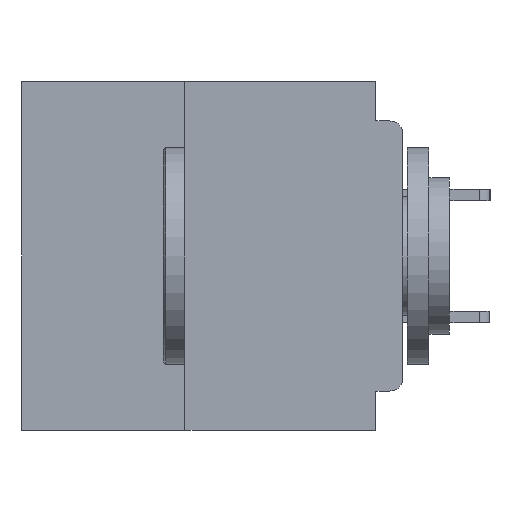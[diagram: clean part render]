
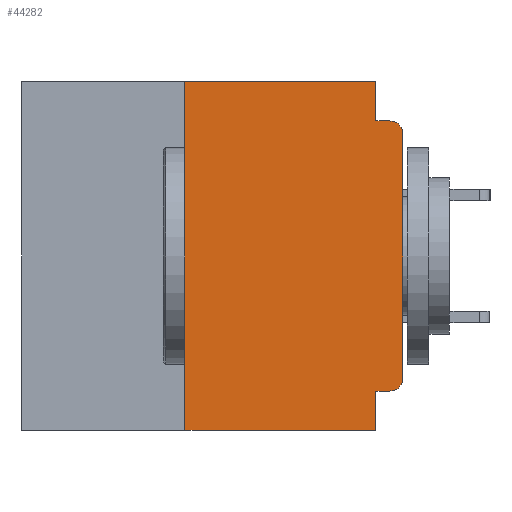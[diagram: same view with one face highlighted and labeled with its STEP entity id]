
A CAD part, left-side view. The second image highlights one B-rep face of the part: STEP entity #44282.
In plain terms, the highlighted planar face has unit normal (-1, 0, 0).
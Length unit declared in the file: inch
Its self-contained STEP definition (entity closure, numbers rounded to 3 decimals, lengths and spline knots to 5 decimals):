
#142 = CARTESIAN_POINT ( 'NONE',  ( 0., 0.031, -0.4 ) ) ;
#254 = CARTESIAN_POINT ( 'NONE',  ( 0., 0., -0.355 ) ) ;
#1671 = VECTOR ( 'NONE', #31259, 39.37008 ) ;
#1722 = LINE ( 'NONE', #44877, #25280 ) ;
#1834 = ORIENTED_EDGE ( 'NONE', *, *, #27117, .F. ) ;
#2905 = DIRECTION ( 'NONE',  ( -1., 0., 0. ) ) ;
#3507 = LINE ( 'NONE', #12196, #28640 ) ;
#3594 = CARTESIAN_POINT ( 'NONE',  ( 0., 0., 0. ) ) ;
#4801 = LINE ( 'NONE', #56178, #1671 ) ;
#7095 = CARTESIAN_POINT ( 'NONE',  ( 0., 0., -0.045 ) ) ;
#7521 = DIRECTION ( 'NONE',  ( 0., -1., 0. ) ) ;
#10218 = VERTEX_POINT ( 'NONE', #39901 ) ;
#11951 = ORIENTED_EDGE ( 'NONE', *, *, #59391, .T. ) ;
#12120 = LINE ( 'NONE', #20560, #50505 ) ;
#12196 = CARTESIAN_POINT ( 'NONE',  ( 0., 0.031, -0.4 ) ) ;
#12401 = CIRCLE ( 'NONE', #51283, 0.015 ) ;
#14349 = EDGE_CURVE ( 'NONE', #18761, #63500, #1722, .T. ) ;
#15446 = DIRECTION ( 'NONE',  ( 1., 0., 0. ) ) ;
#15535 = DIRECTION ( 'NONE',  ( 0., -1., 0. ) ) ;
#16565 = ORIENTED_EDGE ( 'NONE', *, *, #52209, .T. ) ;
#17229 = DIRECTION ( 'NONE',  ( 0., -1., 0. ) ) ;
#17236 = DIRECTION ( 'NONE',  ( 0., 0., -1. ) ) ;
#17350 = CIRCLE ( 'NONE', #60182, 0.015 ) ;
#17466 = FACE_OUTER_BOUND ( 'NONE', #23378, .T. ) ;
#18075 = VERTEX_POINT ( 'NONE', #24660 ) ;
#18497 = VECTOR ( 'NONE', #17229, 39.37008 ) ;
#18761 = VERTEX_POINT ( 'NONE', #25858 ) ;
#19036 = CARTESIAN_POINT ( 'NONE',  ( 0., 0., -0.34 ) ) ;
#20560 = CARTESIAN_POINT ( 'NONE',  ( 0., 0.437, -0.4 ) ) ;
#21001 = CARTESIAN_POINT ( 'NONE',  ( 0., 0.015, -0.06 ) ) ;
#22813 = VERTEX_POINT ( 'NONE', #32500 ) ;
#23378 = EDGE_LOOP ( 'NONE', ( #39533, #40731, #53599, #49705, #42236, #1834, #11951, #56199, #43870, #16565 ) ) ;
#24660 = CARTESIAN_POINT ( 'NONE',  ( 0., 0.25, -0.4 ) ) ;
#24862 = EDGE_CURVE ( 'NONE', #63500, #22813, #33412, .T. ) ;
#25280 = VECTOR ( 'NONE', #29947, 39.37008 ) ;
#25689 = CARTESIAN_POINT ( 'NONE',  ( 0., 0., -0.06 ) ) ;
#25858 = CARTESIAN_POINT ( 'NONE',  ( 0., 0.031, 0. ) ) ;
#26053 = DIRECTION ( 'NONE',  ( 0., 0., -1. ) ) ;
#26804 = CARTESIAN_POINT ( 'NONE',  ( 0., 0.25, 0. ) ) ;
#27117 = EDGE_CURVE ( 'NONE', #18075, #57961, #4801, .T. ) ;
#28640 = VECTOR ( 'NONE', #17236, 39.37008 ) ;
#28821 = DIRECTION ( 'NONE',  ( 0., 0., 1. ) ) ;
#29947 = DIRECTION ( 'NONE',  ( 0., 0., -1. ) ) ;
#31259 = DIRECTION ( 'NONE',  ( 0., 0., 1. ) ) ;
#31350 = VERTEX_POINT ( 'NONE', #19036 ) ;
#31920 = EDGE_CURVE ( 'NONE', #31350, #52558, #50338, .T. ) ;
#32500 = CARTESIAN_POINT ( 'NONE',  ( 0., 0.015, -0.045 ) ) ;
#32507 = CARTESIAN_POINT ( 'NONE',  ( 0., 0.437, 0. ) ) ;
#32633 = VERTEX_POINT ( 'NONE', #54981 ) ;
#32656 = EDGE_CURVE ( 'NONE', #10218, #32633, #59577, .T. ) ;
#32967 = CARTESIAN_POINT ( 'NONE',  ( 0., 0.015, -0.34 ) ) ;
#33412 = LINE ( 'NONE', #7095, #18497 ) ;
#34037 = VECTOR ( 'NONE', #7521, 39.37008 ) ;
#35377 = PLANE ( 'NONE',  #48294 ) ;
#37018 = VECTOR ( 'NONE', #28821, 39.37008 ) ;
#37120 = EDGE_CURVE ( 'NONE', #32633, #58378, #3507, .T. ) ;
#38001 = DIRECTION ( 'NONE',  ( 0., 0., -1. ) ) ;
#39533 = ORIENTED_EDGE ( 'NONE', *, *, #31920, .T. ) ;
#39901 = CARTESIAN_POINT ( 'NONE',  ( 0., 0.015, -0.355 ) ) ;
#40153 = EDGE_CURVE ( 'NONE', #52558, #22813, #17350, .T. ) ;
#40441 = CARTESIAN_POINT ( 'NONE',  ( 0., 0.437, 0. ) ) ;
#40731 = ORIENTED_EDGE ( 'NONE', *, *, #40153, .T. ) ;
#42236 = ORIENTED_EDGE ( 'NONE', *, *, #64357, .F. ) ;
#43870 = ORIENTED_EDGE ( 'NONE', *, *, #32656, .F. ) ;
#44282 = ADVANCED_FACE ( 'NONE', ( #17466 ), #35377, .F. ) ;
#44877 = CARTESIAN_POINT ( 'NONE',  ( 0., 0.031, 0. ) ) ;
#45426 = DIRECTION ( 'NONE',  ( 0., 1., 0. ) ) ;
#48294 = AXIS2_PLACEMENT_3D ( 'NONE', #40441, #15446, #50481 ) ;
#49705 = ORIENTED_EDGE ( 'NONE', *, *, #14349, .F. ) ;
#50338 = LINE ( 'NONE', #3594, #37018 ) ;
#50481 = DIRECTION ( 'NONE',  ( 0., 0., -1. ) ) ;
#50505 = VECTOR ( 'NONE', #15535, 39.37008 ) ;
#51283 = AXIS2_PLACEMENT_3D ( 'NONE', #32967, #2905, #38001 ) ;
#52209 = EDGE_CURVE ( 'NONE', #10218, #31350, #12401, .T. ) ;
#52558 = VERTEX_POINT ( 'NONE', #25689 ) ;
#53599 = ORIENTED_EDGE ( 'NONE', *, *, #24862, .F. ) ;
#54981 = CARTESIAN_POINT ( 'NONE',  ( 0., 0.031, -0.355 ) ) ;
#55998 = DIRECTION ( 'NONE',  ( -1., 0., 0. ) ) ;
#56178 = CARTESIAN_POINT ( 'NONE',  ( 0., 0.25, -0.4 ) ) ;
#56199 = ORIENTED_EDGE ( 'NONE', *, *, #37120, .F. ) ;
#57961 = VERTEX_POINT ( 'NONE', #26804 ) ;
#58022 = VECTOR ( 'NONE', #45426, 39.37008 ) ;
#58378 = VERTEX_POINT ( 'NONE', #142 ) ;
#59391 = EDGE_CURVE ( 'NONE', #18075, #58378, #12120, .T. ) ;
#59577 = LINE ( 'NONE', #254, #58022 ) ;
#60182 = AXIS2_PLACEMENT_3D ( 'NONE', #21001, #55998, #26053 ) ;
#60357 = CARTESIAN_POINT ( 'NONE',  ( 0., 0.031, -0.045 ) ) ;
#62158 = LINE ( 'NONE', #32507, #34037 ) ;
#63500 = VERTEX_POINT ( 'NONE', #60357 ) ;
#64357 = EDGE_CURVE ( 'NONE', #57961, #18761, #62158, .T. ) ;
